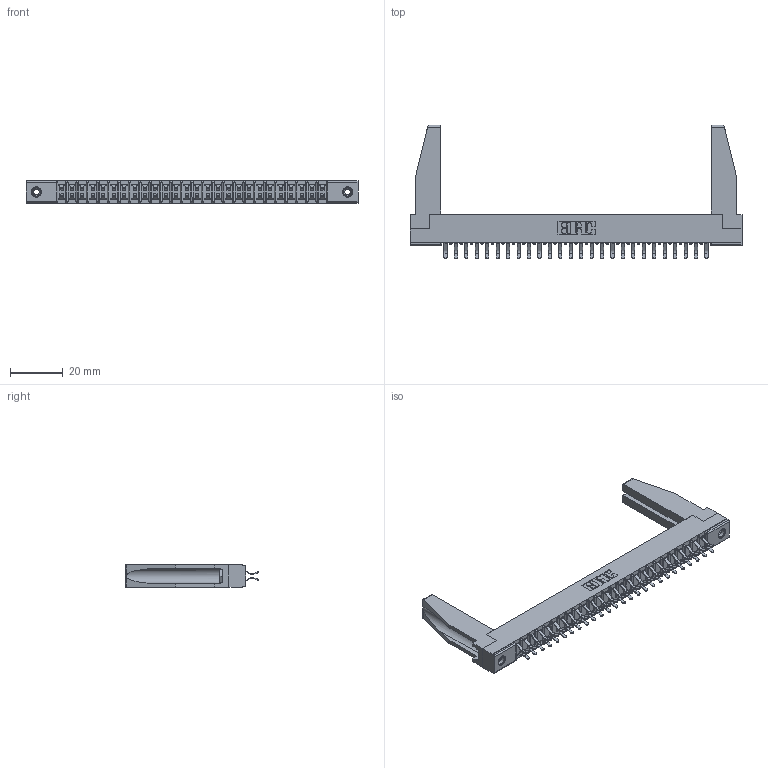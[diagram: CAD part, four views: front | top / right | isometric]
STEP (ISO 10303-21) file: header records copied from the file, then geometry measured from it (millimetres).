
FILE_DESCRIPTION (( 'STEP AP203' ), '1' );
FILE_NAME ('357-052-556-278.STEP', '2019-09-19T03:34:00', ( '' ), ( '' ), 'SwSTEP 2.0', 'SolidWorks 2016', '' );
FILE_SCHEMA (( 'CONFIG_CONTROL_DESIGN' ));
Length unit declared in the file: inch
Products named in the file (5): 307 Part_.156 Dia Mounting Holes; 345-250-001_345-250-001-102; 307-290-001_556; 307-220-078; 357-052-556-278
Assembly tree (57 placements, depth 2):
  357-052-556-278
    307 Part_.156 Dia Mounting Holes
    307-290-001_556  x52
    307-220-078  x2
    345-250-001_345-250-001-102  x2
Bounding box: 126.03 x 50.67 x 8.71 mm (x, y, z)
Volume: 12227.5 mm3; surface area: 18524.2 mm2
Topology: 57 solids, 57 shells, 2875 faces, 8037 edges, 5206 vertices
Faces by surface type: plane 1870, cylinder 935, sphere 54, cone 12, torus 4
Entity records: 27637 total; most frequent: CARTESIAN_POINT 4536, ORIENTED_EDGE 4452, DIRECTION 4404, EDGE_CURVE 2226, VECTOR 1704, LINE 1704, VERTEX_POINT 1440, AXIS2_PLACEMENT_3D 1350
